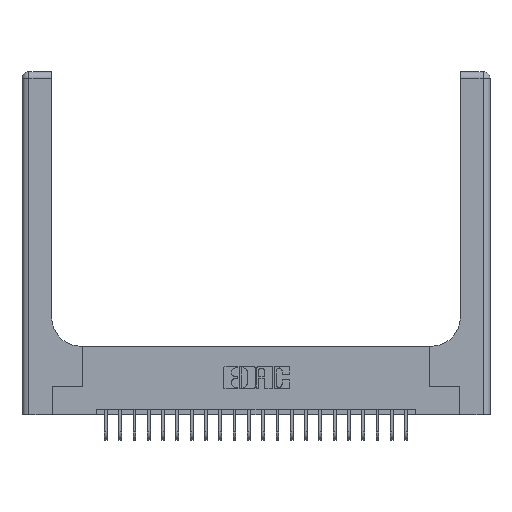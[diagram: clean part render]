
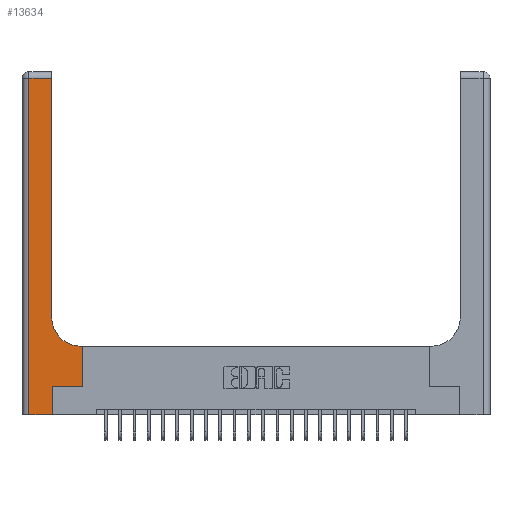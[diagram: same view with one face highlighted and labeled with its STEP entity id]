
A CAD part, top view. The second image highlights one B-rep face of the part: STEP entity #13634.
In plain terms, the highlighted planar face has unit normal (0, 0, 1).
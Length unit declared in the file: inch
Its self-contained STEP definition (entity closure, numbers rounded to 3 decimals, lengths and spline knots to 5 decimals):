
#160 = VECTOR ( 'NONE', #22640, 39.37008 ) ;
#406 = CARTESIAN_POINT ( 'NONE',  ( 0.06, 2.94, 0.37 ) ) ;
#987 = DIRECTION ( 'NONE',  ( 1., 0., 0. ) ) ;
#1366 = VERTEX_POINT ( 'NONE', #2265 ) ;
#1672 = FACE_OUTER_BOUND ( 'NONE', #5355, .T. ) ;
#1714 = AXIS2_PLACEMENT_3D ( 'NONE', #18754, #18872, #15176 ) ;
#2115 = VERTEX_POINT ( 'NONE', #9739 ) ;
#2155 = DIRECTION ( 'NONE',  ( -1., 0., 0. ) ) ;
#2265 = CARTESIAN_POINT ( 'NONE',  ( 0.26, 2.94, 0.37 ) ) ;
#2447 = CIRCLE ( 'NONE', #12325, 0.25 ) ;
#2709 = EDGE_CURVE ( 'NONE', #14689, #2115, #21090, .T. ) ;
#2786 = ORIENTED_EDGE ( 'NONE', *, *, #21651, .T. ) ;
#2837 = VECTOR ( 'NONE', #18095, 39.37008 ) ;
#3091 = CARTESIAN_POINT ( 'NONE',  ( 0.26, 3., 0.37 ) ) ;
#3264 = VECTOR ( 'NONE', #2155, 39.37008 ) ;
#3636 = CARTESIAN_POINT ( 'NONE',  ( 0.51, 0.6, 0.37 ) ) ;
#4019 = LINE ( 'NONE', #11569, #3264 ) ;
#4060 = ORIENTED_EDGE ( 'NONE', *, *, #23889, .T. ) ;
#4202 = EDGE_CURVE ( 'NONE', #2115, #6585, #8671, .T. ) ;
#4472 = VERTEX_POINT ( 'NONE', #12002 ) ;
#4627 = CARTESIAN_POINT ( 'NONE',  ( 0.06, 3., 0.37 ) ) ;
#5294 = ORIENTED_EDGE ( 'NONE', *, *, #22028, .T. ) ;
#5355 = EDGE_LOOP ( 'NONE', ( #19552, #8445, #5294, #22720, #5659, #11361, #4060, #18117, #2786 ) ) ;
#5659 = ORIENTED_EDGE ( 'NONE', *, *, #2709, .T. ) ;
#6585 = VERTEX_POINT ( 'NONE', #10648 ) ;
#7252 = PLANE ( 'NONE',  #1714 ) ;
#7424 = CARTESIAN_POINT ( 'NONE',  ( 0.528, 0.25, 0.37 ) ) ;
#7834 = EDGE_CURVE ( 'NONE', #19460, #1366, #24134, .T. ) ;
#8445 = ORIENTED_EDGE ( 'NONE', *, *, #22508, .T. ) ;
#8671 = LINE ( 'NONE', #22016, #20916 ) ;
#8768 = LINE ( 'NONE', #19772, #22259 ) ;
#9073 = VERTEX_POINT ( 'NONE', #13894 ) ;
#9392 = CARTESIAN_POINT ( 'NONE',  ( 0.26, 0.85, 0.37 ) ) ;
#9393 = VECTOR ( 'NONE', #21448, 39.37008 ) ;
#9739 = CARTESIAN_POINT ( 'NONE',  ( 0.265, 0.25, 0.37 ) ) ;
#10409 = DIRECTION ( 'NONE',  ( -1., 0., 0. ) ) ;
#10648 = CARTESIAN_POINT ( 'NONE',  ( 0.528, 0.25, 0.37 ) ) ;
#11361 = ORIENTED_EDGE ( 'NONE', *, *, #4202, .T. ) ;
#11569 = CARTESIAN_POINT ( 'NONE',  ( 0.26, 0.6, 0.37 ) ) ;
#11572 = VECTOR ( 'NONE', #10409, 39.37008 ) ;
#12002 = CARTESIAN_POINT ( 'NONE',  ( 0.06, 0., 0.37 ) ) ;
#12233 = DIRECTION ( 'NONE',  ( 1., 0., 0. ) ) ;
#12325 = AXIS2_PLACEMENT_3D ( 'NONE', #18614, #14902, #14786 ) ;
#12498 = LINE ( 'NONE', #19794, #11572 ) ;
#13077 = EDGE_CURVE ( 'NONE', #4472, #14689, #8768, .T. ) ;
#13634 = ADVANCED_FACE ( 'NONE', ( #1672 ), #7252, .F. ) ;
#13894 = CARTESIAN_POINT ( 'NONE',  ( 0.528, 0.6, 0.37 ) ) ;
#14689 = VERTEX_POINT ( 'NONE', #22605 ) ;
#14786 = DIRECTION ( 'NONE',  ( 1., 0., 0. ) ) ;
#14902 = DIRECTION ( 'NONE',  ( 0., 0., -1. ) ) ;
#15176 = DIRECTION ( 'NONE',  ( -1., 0., 0. ) ) ;
#15523 = CARTESIAN_POINT ( 'NONE',  ( 0.265, 0., 0.37 ) ) ;
#18081 = DIRECTION ( 'NONE',  ( 0., 1., 0. ) ) ;
#18095 = DIRECTION ( 'NONE',  ( 0., -1., 0. ) ) ;
#18117 = ORIENTED_EDGE ( 'NONE', *, *, #23306, .T. ) ;
#18614 = CARTESIAN_POINT ( 'NONE',  ( 0.51, 0.85, 0.37 ) ) ;
#18754 = CARTESIAN_POINT ( 'NONE',  ( 0., 3., 0.37 ) ) ;
#18872 = DIRECTION ( 'NONE',  ( 0., 0., -1. ) ) ;
#19147 = VERTEX_POINT ( 'NONE', #3636 ) ;
#19460 = VERTEX_POINT ( 'NONE', #9392 ) ;
#19552 = ORIENTED_EDGE ( 'NONE', *, *, #7834, .T. ) ;
#19772 = CARTESIAN_POINT ( 'NONE',  ( 0., 0., 0.37 ) ) ;
#19794 = CARTESIAN_POINT ( 'NONE',  ( 0., 2.94, 0.37 ) ) ;
#20155 = VECTOR ( 'NONE', #18081, 39.37008 ) ;
#20786 = LINE ( 'NONE', #7424, #160 ) ;
#20916 = VECTOR ( 'NONE', #987, 39.37008 ) ;
#21090 = LINE ( 'NONE', #15523, #9393 ) ;
#21448 = DIRECTION ( 'NONE',  ( 0., 1., 0. ) ) ;
#21561 = LINE ( 'NONE', #4627, #2837 ) ;
#21651 = EDGE_CURVE ( 'NONE', #19147, #19460, #2447, .T. ) ;
#21750 = VERTEX_POINT ( 'NONE', #406 ) ;
#22016 = CARTESIAN_POINT ( 'NONE',  ( 0.265, 0.25, 0.37 ) ) ;
#22028 = EDGE_CURVE ( 'NONE', #21750, #4472, #21561, .T. ) ;
#22259 = VECTOR ( 'NONE', #12233, 39.37008 ) ;
#22508 = EDGE_CURVE ( 'NONE', #1366, #21750, #12498, .T. ) ;
#22605 = CARTESIAN_POINT ( 'NONE',  ( 0.265, 0., 0.37 ) ) ;
#22640 = DIRECTION ( 'NONE',  ( 0., 1., 0. ) ) ;
#22720 = ORIENTED_EDGE ( 'NONE', *, *, #13077, .T. ) ;
#23306 = EDGE_CURVE ( 'NONE', #9073, #19147, #4019, .T. ) ;
#23889 = EDGE_CURVE ( 'NONE', #6585, #9073, #20786, .T. ) ;
#24134 = LINE ( 'NONE', #3091, #20155 ) ;
